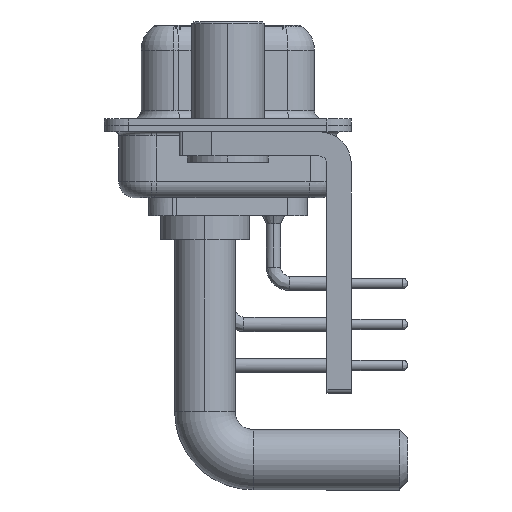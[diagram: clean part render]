
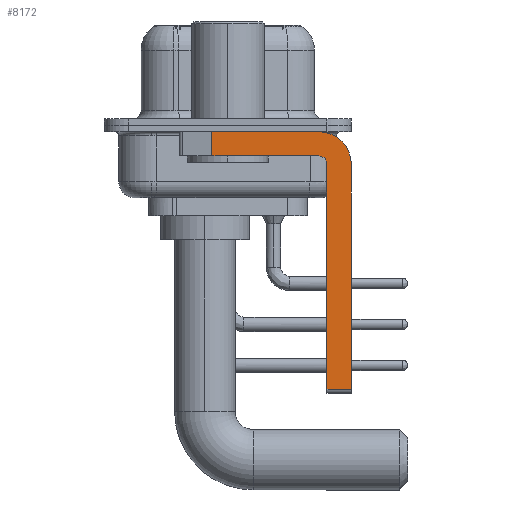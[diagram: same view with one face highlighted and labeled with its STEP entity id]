
A CAD part, left-side view. The second image highlights one B-rep face of the part: STEP entity #8172.
In plain terms, the highlighted planar face has unit normal (-1, 0, 0).
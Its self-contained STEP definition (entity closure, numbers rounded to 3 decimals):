
#759 = AXIS2_PLACEMENT_3D ( 'NONE', #31011, #1211, #27640 ) ;
#1070 = DIRECTION ( 'NONE',  ( 0., 0., -1. ) ) ;
#1211 = DIRECTION ( 'NONE',  ( 1., 0., 0. ) ) ;
#4029 = VECTOR ( 'NONE', #21474, 1000. ) ;
#4171 = CARTESIAN_POINT ( 'NONE',  ( -2.9, -6.15, -16.6 ) ) ;
#4355 = VECTOR ( 'NONE', #29554, 1000. ) ;
#4379 = CARTESIAN_POINT ( 'NONE',  ( -2.9, -6.15, -2.4 ) ) ;
#4655 = ORIENTED_EDGE ( 'NONE', *, *, #27757, .F. ) ;
#5054 = DIRECTION ( 'NONE',  ( 0., -1., 0. ) ) ;
#5065 = ORIENTED_EDGE ( 'NONE', *, *, #19109, .F. ) ;
#5341 = LINE ( 'NONE', #32671, #4029 ) ;
#5382 = CARTESIAN_POINT ( 'NONE',  ( -2.9, 0.978, -1.9 ) ) ;
#5427 = VERTEX_POINT ( 'NONE', #13339 ) ;
#5532 = VERTEX_POINT ( 'NONE', #29140 ) ;
#6092 = VECTOR ( 'NONE', #34502, 1000. ) ;
#6256 = EDGE_CURVE ( 'NONE', #5427, #10545, #5341, .T. ) ;
#6540 = VECTOR ( 'NONE', #14991, 1000. ) ;
#7911 = CARTESIAN_POINT ( 'NONE',  ( -2.9, -5.65, -16.35 ) ) ;
#8172 = ADVANCED_FACE ( 'NONE', ( #25493 ), #20337, .F. ) ;
#8356 = VERTEX_POINT ( 'NONE', #4379 ) ;
#10116 = ORIENTED_EDGE ( 'NONE', *, *, #25344, .T. ) ;
#10208 = ORIENTED_EDGE ( 'NONE', *, *, #18601, .F. ) ;
#10496 = ORIENTED_EDGE ( 'NONE', *, *, #6256, .F. ) ;
#10538 = CARTESIAN_POINT ( 'NONE',  ( -2.9, 3., -0.4 ) ) ;
#10545 = VERTEX_POINT ( 'NONE', #16151 ) ;
#11493 = AXIS2_PLACEMENT_3D ( 'NONE', #13070, #26200, #15372 ) ;
#13070 = CARTESIAN_POINT ( 'NONE',  ( -2.9, -5.65, -2.4 ) ) ;
#13339 = CARTESIAN_POINT ( 'NONE',  ( -2.9, -5.65, -1.9 ) ) ;
#13903 = EDGE_LOOP ( 'NONE', ( #5065, #10116, #10496, #10208, #15791, #20656, #34028, #4655 ) ) ;
#14300 = CARTESIAN_POINT ( 'NONE',  ( -2.9, 0.978, -0.4 ) ) ;
#14520 = LINE ( 'NONE', #17349, #27789 ) ;
#14991 = DIRECTION ( 'NONE',  ( 0., 0., 1. ) ) ;
#15372 = DIRECTION ( 'NONE',  ( 0., 0., 1. ) ) ;
#15475 = CARTESIAN_POINT ( 'NONE',  ( -2.9, -5.65, -2.4 ) ) ;
#15791 = ORIENTED_EDGE ( 'NONE', *, *, #22002, .F. ) ;
#15917 = VERTEX_POINT ( 'NONE', #25920 ) ;
#16035 = CARTESIAN_POINT ( 'NONE',  ( -2.9, -7.65, -16.35 ) ) ;
#16151 = CARTESIAN_POINT ( 'NONE',  ( -2.9, 0.978, -1.9 ) ) ;
#16393 = EDGE_CURVE ( 'NONE', #5532, #30143, #14520, .T. ) ;
#16705 = VERTEX_POINT ( 'NONE', #14300 ) ;
#17120 = VECTOR ( 'NONE', #5054, 1000. ) ;
#17349 = CARTESIAN_POINT ( 'NONE',  ( -2.9, -7.65, -2.4 ) ) ;
#18601 = EDGE_CURVE ( 'NONE', #8356, #5427, #24551, .T. ) ;
#18723 = LINE ( 'NONE', #7911, #4355 ) ;
#19109 = EDGE_CURVE ( 'NONE', #16705, #15917, #20828, .T. ) ;
#20337 = PLANE ( 'NONE',  #759 ) ;
#20656 = ORIENTED_EDGE ( 'NONE', *, *, #24895, .T. ) ;
#20828 = LINE ( 'NONE', #10538, #17120 ) ;
#21474 = DIRECTION ( 'NONE',  ( 0., 1., 0. ) ) ;
#22002 = EDGE_CURVE ( 'NONE', #30353, #8356, #28490, .T. ) ;
#24551 = CIRCLE ( 'NONE', #11493, 0.5 ) ;
#24604 = AXIS2_PLACEMENT_3D ( 'NONE', #15475, #31118, #25601 ) ;
#24895 = EDGE_CURVE ( 'NONE', #30353, #30143, #18723, .T. ) ;
#25344 = EDGE_CURVE ( 'NONE', #16705, #10545, #29167, .T. ) ;
#25493 = FACE_OUTER_BOUND ( 'NONE', #13903, .T. ) ;
#25601 = DIRECTION ( 'NONE',  ( 0., 0., -1. ) ) ;
#25920 = CARTESIAN_POINT ( 'NONE',  ( -2.9, -5.65, -0.4 ) ) ;
#26200 = DIRECTION ( 'NONE',  ( -1., 0., 0. ) ) ;
#27640 = DIRECTION ( 'NONE',  ( 0., 0., -1. ) ) ;
#27757 = EDGE_CURVE ( 'NONE', #15917, #5532, #34848, .T. ) ;
#27789 = VECTOR ( 'NONE', #1070, 1000. ) ;
#28490 = LINE ( 'NONE', #4171, #6540 ) ;
#29140 = CARTESIAN_POINT ( 'NONE',  ( -2.9, -7.65, -2.4 ) ) ;
#29167 = LINE ( 'NONE', #5382, #6092 ) ;
#29554 = DIRECTION ( 'NONE',  ( 0., -1., 0. ) ) ;
#30143 = VERTEX_POINT ( 'NONE', #16035 ) ;
#30353 = VERTEX_POINT ( 'NONE', #30387 ) ;
#30387 = CARTESIAN_POINT ( 'NONE',  ( -2.9, -6.15, -16.35 ) ) ;
#31011 = CARTESIAN_POINT ( 'NONE',  ( -2.9, -5.65, -2.4 ) ) ;
#31118 = DIRECTION ( 'NONE',  ( 1., 0., 0. ) ) ;
#32671 = CARTESIAN_POINT ( 'NONE',  ( -2.9, -5.65, -1.9 ) ) ;
#34028 = ORIENTED_EDGE ( 'NONE', *, *, #16393, .F. ) ;
#34502 = DIRECTION ( 'NONE',  ( 0., 0., -1. ) ) ;
#34848 = CIRCLE ( 'NONE', #24604, 2. ) ;
